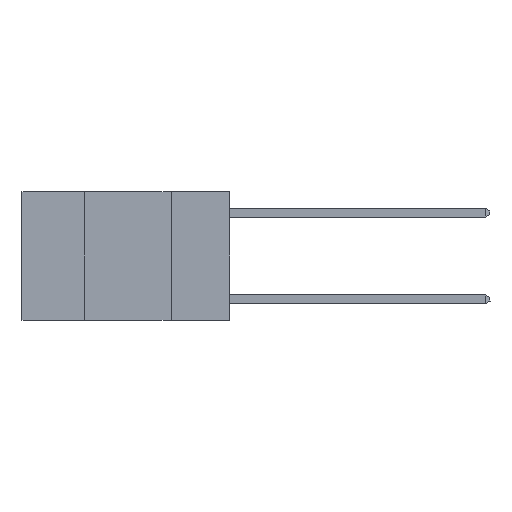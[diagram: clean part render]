
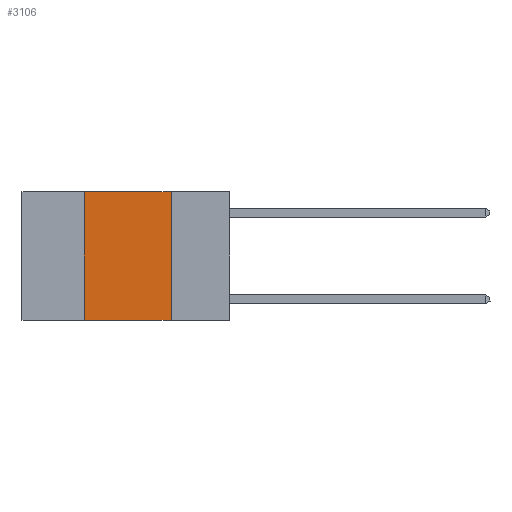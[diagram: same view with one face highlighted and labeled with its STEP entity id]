
A CAD part, left-side view. The second image highlights one B-rep face of the part: STEP entity #3106.
In plain terms, the highlighted planar face has unit normal (-1, 0, 0).
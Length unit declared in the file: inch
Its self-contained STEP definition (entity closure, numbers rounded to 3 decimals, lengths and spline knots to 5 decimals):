
#124 = PLANE ( 'NONE',  #5055 ) ;
#306 = VECTOR ( 'NONE', #8475, 39.37008 ) ;
#328 = CARTESIAN_POINT ( 'NONE',  ( 0., 0.17, 0. ) ) ;
#587 = ORIENTED_EDGE ( 'NONE', *, *, #1717, .F. ) ;
#1288 = VECTOR ( 'NONE', #6324, 39.37008 ) ;
#1561 = ORIENTED_EDGE ( 'NONE', *, *, #5618, .T. ) ;
#1609 = EDGE_CURVE ( 'NONE', #7660, #3397, #7429, .T. ) ;
#1717 = EDGE_CURVE ( 'NONE', #3397, #1968, #2924, .T. ) ;
#1968 = VERTEX_POINT ( 'NONE', #7004 ) ;
#1972 = EDGE_LOOP ( 'NONE', ( #587, #7502, #3432, #1561 ) ) ;
#2200 = VERTEX_POINT ( 'NONE', #6274 ) ;
#2685 = VECTOR ( 'NONE', #4825, 39.37008 ) ;
#2781 = CARTESIAN_POINT ( 'NONE',  ( 0., 0.6, 0. ) ) ;
#2924 = LINE ( 'NONE', #328, #1288 ) ;
#3106 = ADVANCED_FACE ( 'NONE', ( #4201 ), #124, .F. ) ;
#3153 = EDGE_CURVE ( 'NONE', #2200, #7660, #6076, .T. ) ;
#3295 = CARTESIAN_POINT ( 'NONE',  ( 0., 0.17, 0. ) ) ;
#3397 = VERTEX_POINT ( 'NONE', #3295 ) ;
#3432 = ORIENTED_EDGE ( 'NONE', *, *, #3153, .F. ) ;
#3637 = DIRECTION ( 'NONE',  ( 1., 0., 0. ) ) ;
#3773 = VECTOR ( 'NONE', #4411, 39.37008 ) ;
#4201 = FACE_OUTER_BOUND ( 'NONE', #1972, .T. ) ;
#4411 = DIRECTION ( 'NONE',  ( 0., -1., 0. ) ) ;
#4825 = DIRECTION ( 'NONE',  ( 0., -1., 0. ) ) ;
#5002 = CARTESIAN_POINT ( 'NONE',  ( 0., 0.42, 0. ) ) ;
#5055 = AXIS2_PLACEMENT_3D ( 'NONE', #6391, #3637, #8415 ) ;
#5545 = CARTESIAN_POINT ( 'NONE',  ( 0., 0.6, -0.37 ) ) ;
#5618 = EDGE_CURVE ( 'NONE', #2200, #1968, #8138, .T. ) ;
#6076 = LINE ( 'NONE', #7797, #306 ) ;
#6274 = CARTESIAN_POINT ( 'NONE',  ( 0., 0.42, -0.37 ) ) ;
#6324 = DIRECTION ( 'NONE',  ( 0., 0., -1. ) ) ;
#6391 = CARTESIAN_POINT ( 'NONE',  ( 0., 0.6, 0. ) ) ;
#7004 = CARTESIAN_POINT ( 'NONE',  ( 0., 0.17, -0.37 ) ) ;
#7429 = LINE ( 'NONE', #2781, #3773 ) ;
#7502 = ORIENTED_EDGE ( 'NONE', *, *, #1609, .F. ) ;
#7660 = VERTEX_POINT ( 'NONE', #5002 ) ;
#7797 = CARTESIAN_POINT ( 'NONE',  ( 0., 0.42, 0. ) ) ;
#8138 = LINE ( 'NONE', #5545, #2685 ) ;
#8415 = DIRECTION ( 'NONE',  ( 0., 0., -1. ) ) ;
#8475 = DIRECTION ( 'NONE',  ( 0., 0., 1. ) ) ;
